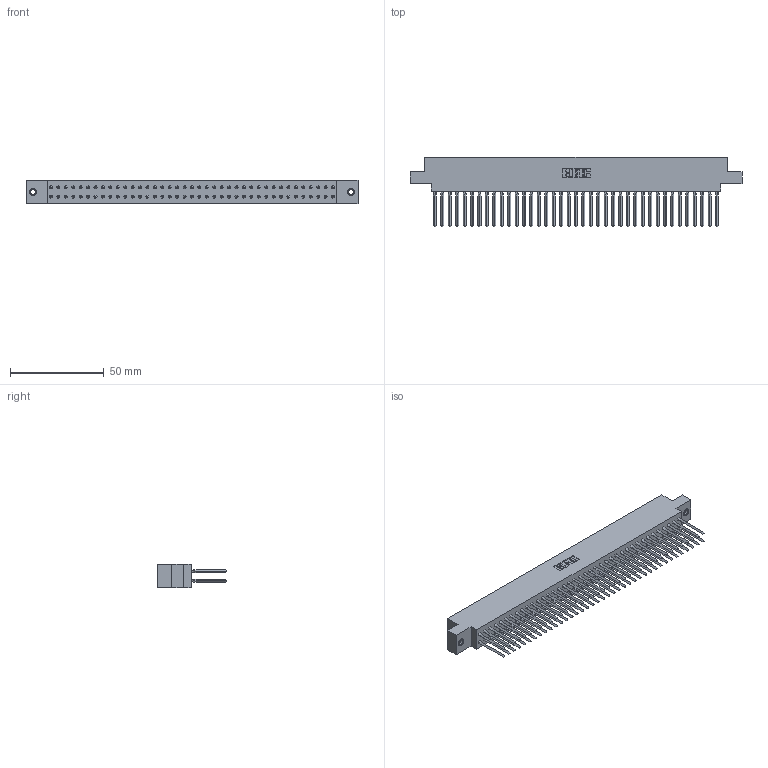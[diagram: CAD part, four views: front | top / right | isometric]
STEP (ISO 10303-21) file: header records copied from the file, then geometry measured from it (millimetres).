
FILE_DESCRIPTION (( 'STEP AP203' ), '1' );
FILE_NAME ('317-078-542-807.STEP', '2020-02-28T08:51:34', ( '' ), ( '' ), 'SwSTEP 2.0', 'SolidWorks 2016', '' );
FILE_SCHEMA (( 'CONFIG_CONTROL_DESIGN' ));
Length unit declared in the file: inch
Products named in the file (4): 345-250-001_345-250-005-103; 317-078-542-807; 317-290-003_542; 317 Part_.156 Dia - TI
Assembly tree (81 placements, depth 2):
  317-078-542-807
    317 Part_.156 Dia - TI
    317-290-003_542  x78
    345-250-001_345-250-005-103  x2
Bounding box: 177.24 x 37.34 x 12.7 mm (x, y, z)
Volume: 28914.3 mm3; surface area: 40148.1 mm2
Topology: 81 solids, 81 shells, 4608 faces, 12891 edges, 8222 vertices
Faces by surface type: plane 3678, cylinder 602, bspline 312, cone 12, torus 4
Entity records: 56996 total; most frequent: CARTESIAN_POINT 10164, ORIENTED_EDGE 9820, DIRECTION 8304, EDGE_CURVE 4910, LINE 4720, VECTOR 4720, VERTEX_POINT 3264, AXIS2_PLACEMENT_3D 1792
